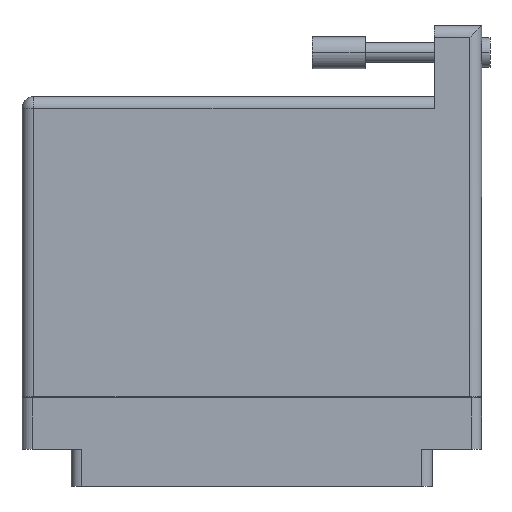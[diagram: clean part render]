
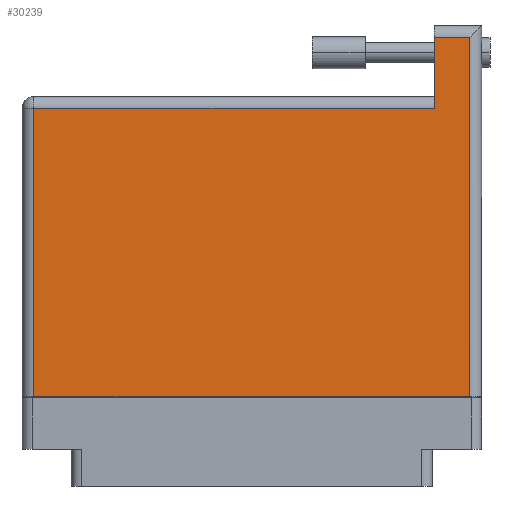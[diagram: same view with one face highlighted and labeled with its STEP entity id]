
A CAD part, front view. The second image highlights one B-rep face of the part: STEP entity #30239.
In plain terms, the highlighted face is planar.
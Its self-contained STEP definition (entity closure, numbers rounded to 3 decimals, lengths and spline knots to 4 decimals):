
#456 = ORIENTED_EDGE ( 'NONE', *, *, #39531, .T. ) ;
#744 = VECTOR ( 'NONE', #62440, 39.3701 ) ;
#1073 = DIRECTION ( 'NONE',  ( 0., 1., 0. ) ) ;
#3494 = CARTESIAN_POINT ( 'NONE',  ( 1.079, 2.025, 0.617 ) ) ;
#6378 = DIRECTION ( 'NONE',  ( -1., 0., 0. ) ) ;
#6644 = EDGE_CURVE ( 'NONE', #19842, #66191, #41759, .T. ) ;
#7857 = DIRECTION ( 'NONE',  ( -1., 0., 0. ) ) ;
#8998 = EDGE_LOOP ( 'NONE', ( #456, #45475, #54305, #53943, #15296, #48404 ) ) ;
#11899 = CARTESIAN_POINT ( 'NONE',  ( 1.079, 1.605, 0.617 ) ) ;
#13035 = VECTOR ( 'NONE', #17565, 39.3701 ) ;
#15108 = AXIS2_PLACEMENT_3D ( 'NONE', #22290, #27514, #6378 ) ;
#15296 = ORIENTED_EDGE ( 'NONE', *, *, #16425, .T. ) ;
#16333 = LINE ( 'NONE', #43794, #13035 ) ;
#16425 = EDGE_CURVE ( 'NONE', #47661, #19842, #16333, .T. ) ;
#17565 = DIRECTION ( 'NONE',  ( -1., 0., 0. ) ) ;
#19842 = VERTEX_POINT ( 'NONE', #3494 ) ;
#20468 = CARTESIAN_POINT ( 'NONE',  ( -1.359, -0.1, 0.617 ) ) ;
#22290 = CARTESIAN_POINT ( 'NONE',  ( -1.359, 1.675, 0.617 ) ) ;
#22920 = LINE ( 'NONE', #66207, #27786 ) ;
#22981 = EDGE_CURVE ( 'NONE', #32728, #47661, #64805, .T. ) ;
#23393 = FACE_OUTER_BOUND ( 'NONE', #8998, .T. ) ;
#23606 = EDGE_CURVE ( 'NONE', #44210, #32728, #52501, .T. ) ;
#23752 = CARTESIAN_POINT ( 'NONE',  ( -1.359, 1.605, 0.617 ) ) ;
#27287 = PLANE ( 'NONE',  #15108 ) ;
#27514 = DIRECTION ( 'NONE',  ( 0., 0., -1. ) ) ;
#27786 = VECTOR ( 'NONE', #66423, 39.3701 ) ;
#28957 = LINE ( 'NONE', #23752, #56152 ) ;
#30239 = ADVANCED_FACE ( 'NONE', ( #23393 ), #27287, .F. ) ;
#32313 = CARTESIAN_POINT ( 'NONE',  ( 1.289, 2.095, 0.617 ) ) ;
#32728 = VERTEX_POINT ( 'NONE', #48091 ) ;
#39531 = EDGE_CURVE ( 'NONE', #66191, #60665, #28957, .T. ) ;
#41759 = LINE ( 'NONE', #42509, #45902 ) ;
#41975 = CARTESIAN_POINT ( 'NONE',  ( -1.289, -0.1, 0.617 ) ) ;
#42509 = CARTESIAN_POINT ( 'NONE',  ( 1.079, 2.095, 0.617 ) ) ;
#43444 = DIRECTION ( 'NONE',  ( 0., -1., 0. ) ) ;
#43794 = CARTESIAN_POINT ( 'NONE',  ( -1.359, 2.025, 0.617 ) ) ;
#44210 = VERTEX_POINT ( 'NONE', #41975 ) ;
#44309 = VECTOR ( 'NONE', #1073, 39.3701 ) ;
#45475 = ORIENTED_EDGE ( 'NONE', *, *, #52079, .T. ) ;
#45902 = VECTOR ( 'NONE', #43444, 39.3701 ) ;
#47661 = VERTEX_POINT ( 'NONE', #65523 ) ;
#48091 = CARTESIAN_POINT ( 'NONE',  ( 1.289, -0.1, 0.617 ) ) ;
#48404 = ORIENTED_EDGE ( 'NONE', *, *, #6644, .T. ) ;
#49647 = CARTESIAN_POINT ( 'NONE',  ( -1.289, 1.605, 0.617 ) ) ;
#52079 = EDGE_CURVE ( 'NONE', #60665, #44210, #22920, .T. ) ;
#52501 = LINE ( 'NONE', #20468, #744 ) ;
#53943 = ORIENTED_EDGE ( 'NONE', *, *, #22981, .T. ) ;
#54305 = ORIENTED_EDGE ( 'NONE', *, *, #23606, .T. ) ;
#56152 = VECTOR ( 'NONE', #7857, 39.3701 ) ;
#60665 = VERTEX_POINT ( 'NONE', #49647 ) ;
#62440 = DIRECTION ( 'NONE',  ( 1., 0., 0. ) ) ;
#64805 = LINE ( 'NONE', #32313, #44309 ) ;
#65523 = CARTESIAN_POINT ( 'NONE',  ( 1.289, 2.025, 0.617 ) ) ;
#66191 = VERTEX_POINT ( 'NONE', #11899 ) ;
#66207 = CARTESIAN_POINT ( 'NONE',  ( -1.289, -0.1, 0.617 ) ) ;
#66423 = DIRECTION ( 'NONE',  ( 0., -1., 0. ) ) ;
